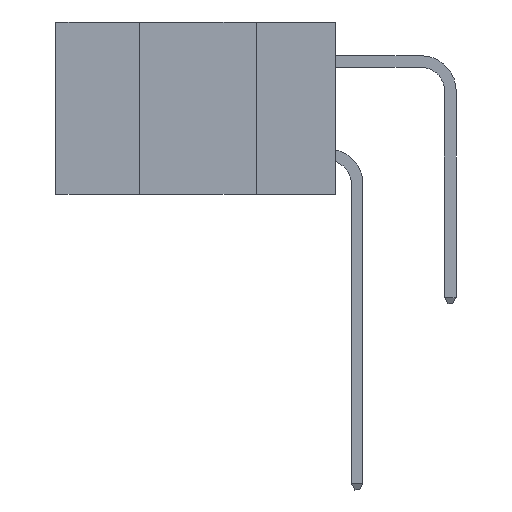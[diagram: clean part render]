
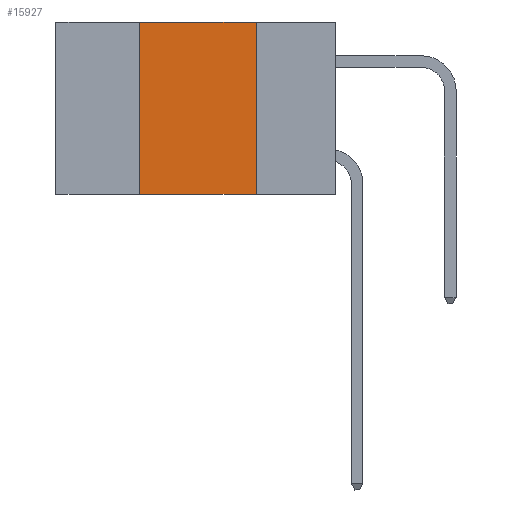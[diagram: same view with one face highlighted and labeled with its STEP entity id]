
A CAD part, left-side view. The second image highlights one B-rep face of the part: STEP entity #15927.
In plain terms, the highlighted planar face has unit normal (-1, 0, 0).
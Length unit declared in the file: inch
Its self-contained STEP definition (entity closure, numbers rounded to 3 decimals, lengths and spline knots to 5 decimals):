
#76 = DIRECTION ( 'NONE',  ( 0., 0., -1. ) ) ;
#142 = AXIS2_PLACEMENT_3D ( 'NONE', #6188, #7496, #3690 ) ;
#1045 = PLANE ( 'NONE',  #142 ) ;
#1704 = EDGE_CURVE ( 'NONE', #2624, #10617, #7129, .T. ) ;
#2215 = VECTOR ( 'NONE', #14897, 39.37008 ) ;
#2278 = LINE ( 'NONE', #7084, #15891 ) ;
#2624 = VERTEX_POINT ( 'NONE', #4526 ) ;
#2959 = VECTOR ( 'NONE', #14910, 39.37008 ) ;
#3217 = EDGE_LOOP ( 'NONE', ( #12281, #7714, #12538, #12712 ) ) ;
#3690 = DIRECTION ( 'NONE',  ( 0., 0., -1. ) ) ;
#4526 = CARTESIAN_POINT ( 'NONE',  ( 0., 0.17, 0. ) ) ;
#4581 = LINE ( 'NONE', #5908, #2959 ) ;
#5770 = CARTESIAN_POINT ( 'NONE',  ( 0., 0.42, -0.37 ) ) ;
#5908 = CARTESIAN_POINT ( 'NONE',  ( 0., 0.6, 0. ) ) ;
#6188 = CARTESIAN_POINT ( 'NONE',  ( 0., 0.6, 0. ) ) ;
#7084 = CARTESIAN_POINT ( 'NONE',  ( 0., 0.6, -0.37 ) ) ;
#7124 = EDGE_CURVE ( 'NONE', #7550, #10617, #2278, .T. ) ;
#7129 = LINE ( 'NONE', #15430, #14952 ) ;
#7496 = DIRECTION ( 'NONE',  ( 1., 0., 0. ) ) ;
#7550 = VERTEX_POINT ( 'NONE', #5770 ) ;
#7714 = ORIENTED_EDGE ( 'NONE', *, *, #10584, .F. ) ;
#7781 = LINE ( 'NONE', #12102, #2215 ) ;
#8702 = FACE_OUTER_BOUND ( 'NONE', #3217, .T. ) ;
#8742 = EDGE_CURVE ( 'NONE', #7550, #11050, #7781, .T. ) ;
#10584 = EDGE_CURVE ( 'NONE', #11050, #2624, #4581, .T. ) ;
#10617 = VERTEX_POINT ( 'NONE', #14740 ) ;
#11050 = VERTEX_POINT ( 'NONE', #15783 ) ;
#12102 = CARTESIAN_POINT ( 'NONE',  ( 0., 0.42, 0. ) ) ;
#12281 = ORIENTED_EDGE ( 'NONE', *, *, #1704, .F. ) ;
#12538 = ORIENTED_EDGE ( 'NONE', *, *, #8742, .F. ) ;
#12712 = ORIENTED_EDGE ( 'NONE', *, *, #7124, .T. ) ;
#14740 = CARTESIAN_POINT ( 'NONE',  ( 0., 0.17, -0.37 ) ) ;
#14897 = DIRECTION ( 'NONE',  ( 0., 0., 1. ) ) ;
#14910 = DIRECTION ( 'NONE',  ( 0., -1., 0. ) ) ;
#14952 = VECTOR ( 'NONE', #76, 39.37008 ) ;
#15430 = CARTESIAN_POINT ( 'NONE',  ( 0., 0.17, 0. ) ) ;
#15783 = CARTESIAN_POINT ( 'NONE',  ( 0., 0.42, 0. ) ) ;
#15891 = VECTOR ( 'NONE', #16050, 39.37008 ) ;
#15927 = ADVANCED_FACE ( 'NONE', ( #8702 ), #1045, .F. ) ;
#16050 = DIRECTION ( 'NONE',  ( 0., -1., 0. ) ) ;
